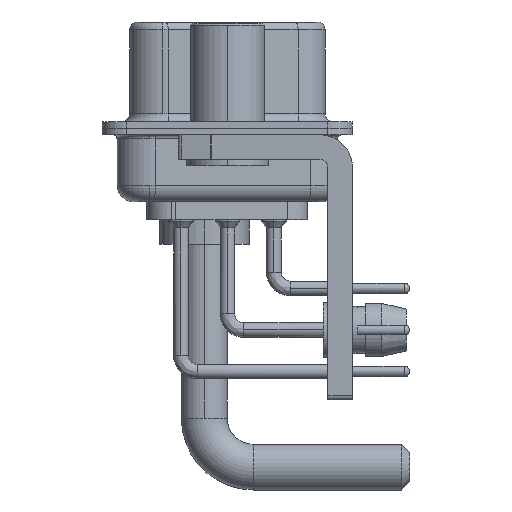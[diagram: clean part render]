
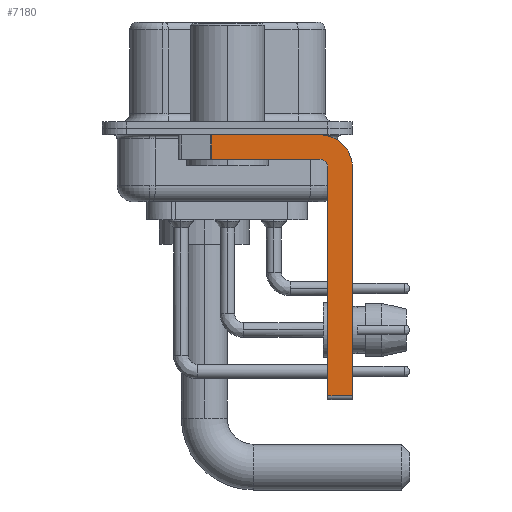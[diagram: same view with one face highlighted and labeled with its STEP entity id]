
A CAD part, left-side view. The second image highlights one B-rep face of the part: STEP entity #7180.
In plain terms, the highlighted planar face has unit normal (-1, 0, 0).
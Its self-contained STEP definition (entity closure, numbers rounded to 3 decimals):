
#12 = CARTESIAN_POINT ( 'NONE',  ( -2.9, -6.15, -2.4 ) ) ;
#883 = DIRECTION ( 'NONE',  ( -1., 0., 0. ) ) ;
#1974 = ORIENTED_EDGE ( 'NONE', *, *, #11461, .F. ) ;
#2329 = CARTESIAN_POINT ( 'NONE',  ( -2.9, 0.978, -0.4 ) ) ;
#2697 = CARTESIAN_POINT ( 'NONE',  ( -2.9, -6.15, -16.35 ) ) ;
#2874 = CARTESIAN_POINT ( 'NONE',  ( -2.9, -7.65, -2.4 ) ) ;
#3049 = VERTEX_POINT ( 'NONE', #2329 ) ;
#3366 = FACE_OUTER_BOUND ( 'NONE', #36340, .T. ) ;
#3469 = VERTEX_POINT ( 'NONE', #30226 ) ;
#5980 = LINE ( 'NONE', #2874, #30531 ) ;
#6376 = CARTESIAN_POINT ( 'NONE',  ( -2.9, -5.65, -1.9 ) ) ;
#7180 = ADVANCED_FACE ( 'NONE', ( #3366 ), #18711, .F. ) ;
#7233 = CARTESIAN_POINT ( 'NONE',  ( -2.9, -6.15, -16.6 ) ) ;
#7421 = EDGE_CURVE ( 'NONE', #16646, #8114, #34438, .T. ) ;
#7434 = VERTEX_POINT ( 'NONE', #13526 ) ;
#8114 = VERTEX_POINT ( 'NONE', #11388 ) ;
#9462 = ORIENTED_EDGE ( 'NONE', *, *, #9520, .F. ) ;
#9520 = EDGE_CURVE ( 'NONE', #40110, #3469, #5980, .T. ) ;
#9616 = CARTESIAN_POINT ( 'NONE',  ( -2.9, -5.65, -2.4 ) ) ;
#11388 = CARTESIAN_POINT ( 'NONE',  ( -2.9, -5.65, -1.9 ) ) ;
#11461 = EDGE_CURVE ( 'NONE', #8114, #7434, #34738, .T. ) ;
#11887 = LINE ( 'NONE', #12103, #31692 ) ;
#12103 = CARTESIAN_POINT ( 'NONE',  ( -2.9, 3., -0.4 ) ) ;
#12491 = CARTESIAN_POINT ( 'NONE',  ( -2.9, 0.978, -1.9 ) ) ;
#12600 = VERTEX_POINT ( 'NONE', #30458 ) ;
#13044 = CIRCLE ( 'NONE', #36184, 2. ) ;
#13526 = CARTESIAN_POINT ( 'NONE',  ( -2.9, 0.978, -1.9 ) ) ;
#15067 = VERTEX_POINT ( 'NONE', #2697 ) ;
#15197 = ORIENTED_EDGE ( 'NONE', *, *, #20835, .F. ) ;
#15452 = CARTESIAN_POINT ( 'NONE',  ( -2.9, -7.65, -2.4 ) ) ;
#16607 = DIRECTION ( 'NONE',  ( 0., -1., 0. ) ) ;
#16646 = VERTEX_POINT ( 'NONE', #12 ) ;
#16690 = ORIENTED_EDGE ( 'NONE', *, *, #17031, .F. ) ;
#17031 = EDGE_CURVE ( 'NONE', #12600, #40110, #13044, .T. ) ;
#18097 = DIRECTION ( 'NONE',  ( 0., -1., 0. ) ) ;
#18711 = PLANE ( 'NONE',  #33066 ) ;
#18998 = DIRECTION ( 'NONE',  ( 0., 1., 0. ) ) ;
#19638 = DIRECTION ( 'NONE',  ( 0., 0., 1. ) ) ;
#20835 = EDGE_CURVE ( 'NONE', #3049, #12600, #11887, .T. ) ;
#22009 = DIRECTION ( 'NONE',  ( 1., 0., 0. ) ) ;
#22595 = LINE ( 'NONE', #26317, #33168 ) ;
#23632 = DIRECTION ( 'NONE',  ( 0., 0., 1. ) ) ;
#24329 = EDGE_CURVE ( 'NONE', #15067, #16646, #36383, .T. ) ;
#25092 = DIRECTION ( 'NONE',  ( 0., 0., -1. ) ) ;
#25523 = DIRECTION ( 'NONE',  ( 0., 0., -1. ) ) ;
#26014 = DIRECTION ( 'NONE',  ( 0., 0., -1. ) ) ;
#26317 = CARTESIAN_POINT ( 'NONE',  ( -2.9, -5.65, -16.35 ) ) ;
#27891 = CARTESIAN_POINT ( 'NONE',  ( -2.9, -5.65, -2.4 ) ) ;
#29807 = AXIS2_PLACEMENT_3D ( 'NONE', #32554, #883, #23632 ) ;
#29886 = VECTOR ( 'NONE', #19638, 1000. ) ;
#30226 = CARTESIAN_POINT ( 'NONE',  ( -2.9, -7.65, -16.35 ) ) ;
#30458 = CARTESIAN_POINT ( 'NONE',  ( -2.9, -5.65, -0.4 ) ) ;
#30531 = VECTOR ( 'NONE', #38062, 1000. ) ;
#31692 = VECTOR ( 'NONE', #18097, 1000. ) ;
#32554 = CARTESIAN_POINT ( 'NONE',  ( -2.9, -5.65, -2.4 ) ) ;
#33021 = ORIENTED_EDGE ( 'NONE', *, *, #7421, .F. ) ;
#33066 = AXIS2_PLACEMENT_3D ( 'NONE', #9616, #22009, #25523 ) ;
#33168 = VECTOR ( 'NONE', #16607, 1000. ) ;
#34265 = EDGE_CURVE ( 'NONE', #15067, #3469, #22595, .T. ) ;
#34436 = ORIENTED_EDGE ( 'NONE', *, *, #24329, .F. ) ;
#34438 = CIRCLE ( 'NONE', #29807, 0.5 ) ;
#34738 = LINE ( 'NONE', #6376, #37272 ) ;
#35328 = DIRECTION ( 'NONE',  ( 1., 0., 0. ) ) ;
#36184 = AXIS2_PLACEMENT_3D ( 'NONE', #27891, #35328, #26014 ) ;
#36340 = EDGE_LOOP ( 'NONE', ( #15197, #39652, #1974, #33021, #34436, #36707, #9462, #16690 ) ) ;
#36383 = LINE ( 'NONE', #7233, #29886 ) ;
#36707 = ORIENTED_EDGE ( 'NONE', *, *, #34265, .T. ) ;
#37272 = VECTOR ( 'NONE', #18998, 1000. ) ;
#37982 = EDGE_CURVE ( 'NONE', #3049, #7434, #40823, .T. ) ;
#38062 = DIRECTION ( 'NONE',  ( 0., 0., -1. ) ) ;
#39652 = ORIENTED_EDGE ( 'NONE', *, *, #37982, .T. ) ;
#40110 = VERTEX_POINT ( 'NONE', #15452 ) ;
#40234 = VECTOR ( 'NONE', #25092, 1000. ) ;
#40823 = LINE ( 'NONE', #12491, #40234 ) ;
